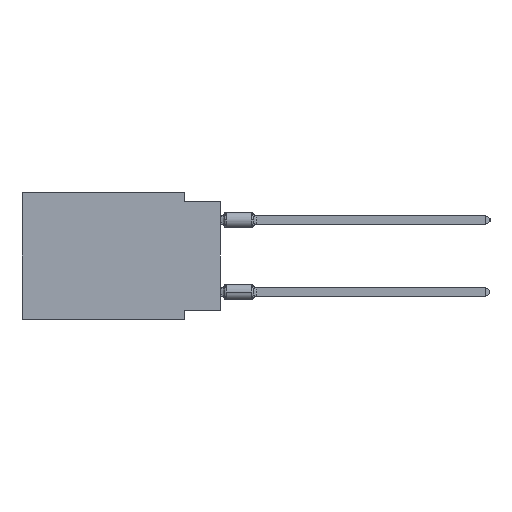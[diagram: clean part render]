
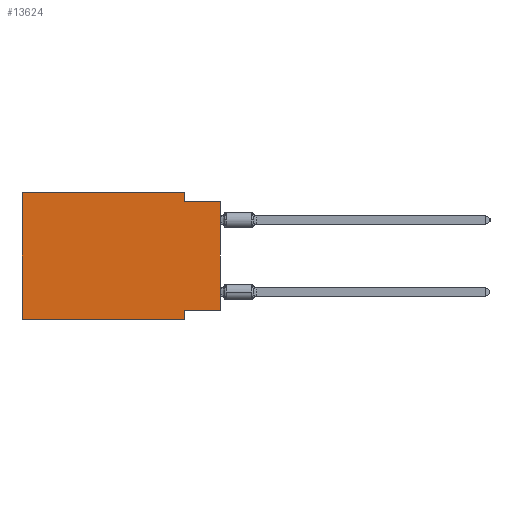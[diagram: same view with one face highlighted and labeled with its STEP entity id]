
A CAD part, left-side view. The second image highlights one B-rep face of the part: STEP entity #13624.
In plain terms, the highlighted planar face has unit normal (-1, 0, 0).
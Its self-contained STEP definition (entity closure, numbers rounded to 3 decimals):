
#87 = DIRECTION ( 'NONE',  ( 0., 0., 1. ) ) ;
#287 = ORIENTED_EDGE ( 'NONE', *, *, #23191, .F. ) ;
#432 = LINE ( 'NONE', #11808, #25827 ) ;
#1556 = CARTESIAN_POINT ( 'NONE',  ( 0., 2.54, -8.89 ) ) ;
#2116 = CARTESIAN_POINT ( 'NONE',  ( 0., 2.54, 0. ) ) ;
#2396 = VECTOR ( 'NONE', #20292, 1000. ) ;
#2840 = LINE ( 'NONE', #22159, #5709 ) ;
#2931 = EDGE_CURVE ( 'NONE', #33398, #14106, #14522, .T. ) ;
#3221 = ORIENTED_EDGE ( 'NONE', *, *, #30182, .F. ) ;
#3681 = FACE_OUTER_BOUND ( 'NONE', #23374, .T. ) ;
#3823 = DIRECTION ( 'NONE',  ( 0., 0., -1. ) ) ;
#5426 = VECTOR ( 'NONE', #9576, 1000. ) ;
#5709 = VECTOR ( 'NONE', #33162, 1000. ) ;
#5737 = VERTEX_POINT ( 'NONE', #10244 ) ;
#6178 = LINE ( 'NONE', #33801, #10260 ) ;
#6470 = LINE ( 'NONE', #14602, #14246 ) ;
#6854 = CARTESIAN_POINT ( 'NONE',  ( 0., 13.97, 0. ) ) ;
#9272 = CARTESIAN_POINT ( 'NONE',  ( 0., 13.97, 0. ) ) ;
#9576 = DIRECTION ( 'NONE',  ( 0., 0., 1. ) ) ;
#10243 = EDGE_CURVE ( 'NONE', #24599, #22910, #26179, .T. ) ;
#10244 = CARTESIAN_POINT ( 'NONE',  ( 0., 2.54, -8.89 ) ) ;
#10260 = VECTOR ( 'NONE', #3823, 1000. ) ;
#11071 = ORIENTED_EDGE ( 'NONE', *, *, #29057, .F. ) ;
#11808 = CARTESIAN_POINT ( 'NONE',  ( 0., 0., 0. ) ) ;
#13189 = EDGE_CURVE ( 'NONE', #24599, #5737, #6470, .T. ) ;
#13624 = ADVANCED_FACE ( 'NONE', ( #3681 ), #25694, .F. ) ;
#13823 = CARTESIAN_POINT ( 'NONE',  ( 0., 13.97, -8.89 ) ) ;
#13932 = VECTOR ( 'NONE', #29004, 1000. ) ;
#14106 = VERTEX_POINT ( 'NONE', #14378 ) ;
#14220 = CARTESIAN_POINT ( 'NONE',  ( 0., 2.54, -8.255 ) ) ;
#14246 = VECTOR ( 'NONE', #25614, 1000. ) ;
#14378 = CARTESIAN_POINT ( 'NONE',  ( 0., 0., -0.635 ) ) ;
#14522 = LINE ( 'NONE', #25539, #2396 ) ;
#14602 = CARTESIAN_POINT ( 'NONE',  ( 0., 13.97, -8.89 ) ) ;
#14712 = CARTESIAN_POINT ( 'NONE',  ( 0., 2.54, -0.635 ) ) ;
#14849 = DIRECTION ( 'NONE',  ( 0., 0., -1. ) ) ;
#15703 = EDGE_CURVE ( 'NONE', #31069, #14106, #432, .T. ) ;
#17582 = DIRECTION ( 'NONE',  ( 1., 0., 0. ) ) ;
#19003 = ORIENTED_EDGE ( 'NONE', *, *, #13189, .T. ) ;
#20292 = DIRECTION ( 'NONE',  ( 0., -1., 0. ) ) ;
#20999 = ORIENTED_EDGE ( 'NONE', *, *, #34904, .F. ) ;
#22159 = CARTESIAN_POINT ( 'NONE',  ( 0., 13.97, 0. ) ) ;
#22910 = VERTEX_POINT ( 'NONE', #35371 ) ;
#23191 = EDGE_CURVE ( 'NONE', #31069, #25407, #28819, .T. ) ;
#23374 = EDGE_LOOP ( 'NONE', ( #34772, #27341, #11071, #3221, #28984, #19003, #20999, #287 ) ) ;
#24599 = VERTEX_POINT ( 'NONE', #13823 ) ;
#25407 = VERTEX_POINT ( 'NONE', #14220 ) ;
#25539 = CARTESIAN_POINT ( 'NONE',  ( 0., 0., -0.635 ) ) ;
#25614 = DIRECTION ( 'NONE',  ( 0., -1., 0. ) ) ;
#25694 = PLANE ( 'NONE',  #26925 ) ;
#25827 = VECTOR ( 'NONE', #87, 1000. ) ;
#25951 = CARTESIAN_POINT ( 'NONE',  ( 0., 0., -8.255 ) ) ;
#26179 = LINE ( 'NONE', #6854, #5426 ) ;
#26468 = CARTESIAN_POINT ( 'NONE',  ( 0., 0., -8.255 ) ) ;
#26925 = AXIS2_PLACEMENT_3D ( 'NONE', #9272, #17582, #14849 ) ;
#27341 = ORIENTED_EDGE ( 'NONE', *, *, #2931, .F. ) ;
#28819 = LINE ( 'NONE', #26468, #29942 ) ;
#28984 = ORIENTED_EDGE ( 'NONE', *, *, #10243, .F. ) ;
#29004 = DIRECTION ( 'NONE',  ( 0., 0., -1. ) ) ;
#29057 = EDGE_CURVE ( 'NONE', #31158, #33398, #6178, .T. ) ;
#29942 = VECTOR ( 'NONE', #31882, 1000. ) ;
#30182 = EDGE_CURVE ( 'NONE', #22910, #31158, #2840, .T. ) ;
#31069 = VERTEX_POINT ( 'NONE', #25951 ) ;
#31158 = VERTEX_POINT ( 'NONE', #2116 ) ;
#31882 = DIRECTION ( 'NONE',  ( 0., 1., 0. ) ) ;
#33162 = DIRECTION ( 'NONE',  ( 0., -1., 0. ) ) ;
#33398 = VERTEX_POINT ( 'NONE', #14712 ) ;
#33801 = CARTESIAN_POINT ( 'NONE',  ( 0., 2.54, 0. ) ) ;
#34772 = ORIENTED_EDGE ( 'NONE', *, *, #15703, .T. ) ;
#34904 = EDGE_CURVE ( 'NONE', #25407, #5737, #34955, .T. ) ;
#34955 = LINE ( 'NONE', #1556, #13932 ) ;
#35371 = CARTESIAN_POINT ( 'NONE',  ( 0., 13.97, 0. ) ) ;
